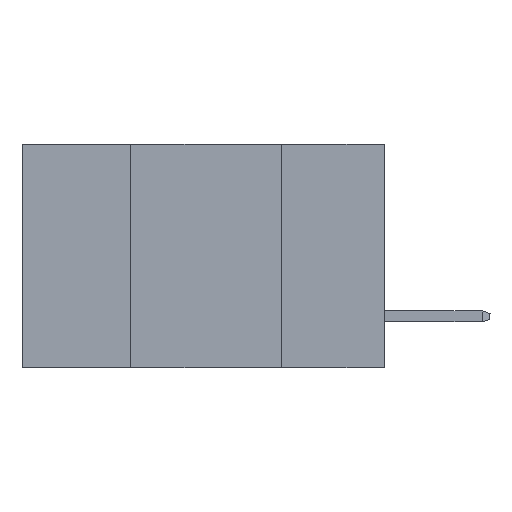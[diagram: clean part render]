
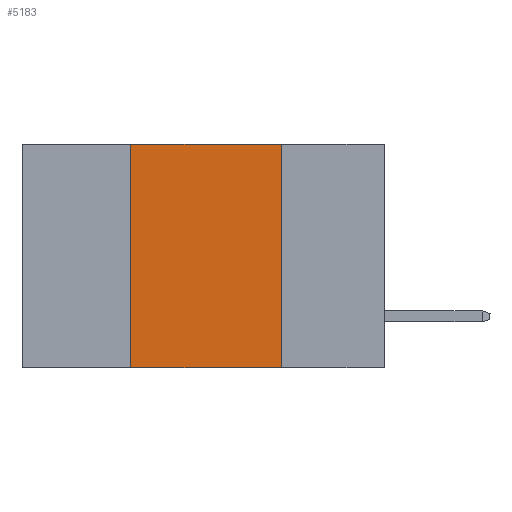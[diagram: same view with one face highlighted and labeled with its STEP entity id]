
A CAD part, left-side view. The second image highlights one B-rep face of the part: STEP entity #5183.
In plain terms, the highlighted planar face has unit normal (-1, 0, 0).
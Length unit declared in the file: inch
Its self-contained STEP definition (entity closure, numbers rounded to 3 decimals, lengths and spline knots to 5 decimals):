
#80 = DIRECTION ( 'NONE',  ( 0., 0., -1. ) ) ;
#619 = EDGE_CURVE ( 'NONE', #4844, #12466, #2725, .T. ) ;
#893 = VECTOR ( 'NONE', #2490, 39.37008 ) ;
#935 = EDGE_CURVE ( 'NONE', #4844, #8522, #2950, .T. ) ;
#1124 = VECTOR ( 'NONE', #3058, 39.37008 ) ;
#1149 = ORIENTED_EDGE ( 'NONE', *, *, #935, .T. ) ;
#1506 = VECTOR ( 'NONE', #10609, 39.37008 ) ;
#2076 = CARTESIAN_POINT ( 'NONE',  ( 0., 0.17, -0.37 ) ) ;
#2158 = CARTESIAN_POINT ( 'NONE',  ( 0., 0.6, -0.37 ) ) ;
#2490 = DIRECTION ( 'NONE',  ( 0., -1., 0. ) ) ;
#2725 = LINE ( 'NONE', #13491, #13113 ) ;
#2950 = LINE ( 'NONE', #2158, #1506 ) ;
#3058 = DIRECTION ( 'NONE',  ( 0., 0., -1. ) ) ;
#3845 = ORIENTED_EDGE ( 'NONE', *, *, #4379, .F. ) ;
#3920 = LINE ( 'NONE', #6164, #1124 ) ;
#4379 = EDGE_CURVE ( 'NONE', #7564, #8522, #3920, .T. ) ;
#4383 = LINE ( 'NONE', #9841, #893 ) ;
#4844 = VERTEX_POINT ( 'NONE', #11821 ) ;
#5183 = ADVANCED_FACE ( 'NONE', ( #8788 ), #6506, .F. ) ;
#5955 = DIRECTION ( 'NONE',  ( 1., 0., 0. ) ) ;
#6164 = CARTESIAN_POINT ( 'NONE',  ( 0., 0.17, -0.37 ) ) ;
#6506 = PLANE ( 'NONE',  #7187 ) ;
#7187 = AXIS2_PLACEMENT_3D ( 'NONE', #12294, #5955, #80 ) ;
#7564 = VERTEX_POINT ( 'NONE', #12343 ) ;
#8522 = VERTEX_POINT ( 'NONE', #2076 ) ;
#8788 = FACE_OUTER_BOUND ( 'NONE', #10638, .T. ) ;
#9841 = CARTESIAN_POINT ( 'NONE',  ( 0., 0.6, 0. ) ) ;
#10609 = DIRECTION ( 'NONE',  ( 0., -1., 0. ) ) ;
#10638 = EDGE_LOOP ( 'NONE', ( #3845, #13317, #12991, #1149 ) ) ;
#10720 = CARTESIAN_POINT ( 'NONE',  ( 0., 0.42, 0. ) ) ;
#11821 = CARTESIAN_POINT ( 'NONE',  ( 0., 0.42, -0.37 ) ) ;
#12294 = CARTESIAN_POINT ( 'NONE',  ( 0., 0.6, 0. ) ) ;
#12343 = CARTESIAN_POINT ( 'NONE',  ( 0., 0.17, 0. ) ) ;
#12466 = VERTEX_POINT ( 'NONE', #10720 ) ;
#12586 = DIRECTION ( 'NONE',  ( 0., 0., 1. ) ) ;
#12991 = ORIENTED_EDGE ( 'NONE', *, *, #619, .F. ) ;
#13113 = VECTOR ( 'NONE', #12586, 39.37008 ) ;
#13317 = ORIENTED_EDGE ( 'NONE', *, *, #13667, .F. ) ;
#13491 = CARTESIAN_POINT ( 'NONE',  ( 0., 0.42, -0.37 ) ) ;
#13667 = EDGE_CURVE ( 'NONE', #12466, #7564, #4383, .T. ) ;
